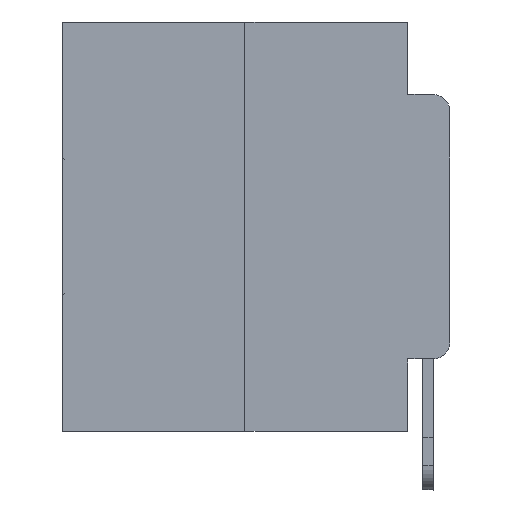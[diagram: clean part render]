
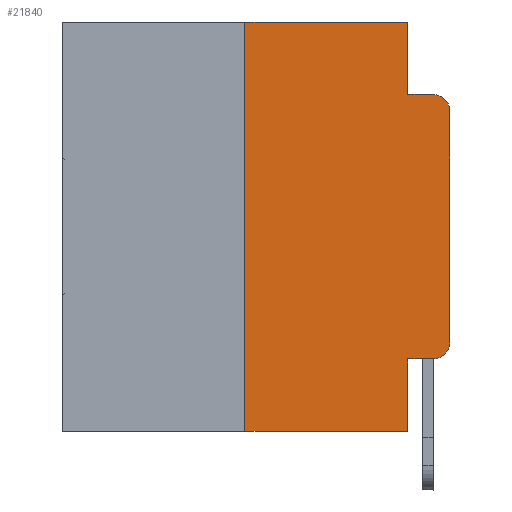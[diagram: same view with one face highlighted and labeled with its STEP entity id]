
A CAD part, left-side view. The second image highlights one B-rep face of the part: STEP entity #21840.
In plain terms, the highlighted planar face has unit normal (-1, 0, 0).
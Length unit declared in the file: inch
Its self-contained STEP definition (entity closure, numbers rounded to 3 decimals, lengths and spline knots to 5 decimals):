
#330 = VECTOR ( 'NONE', #6012, 39.37008 ) ;
#424 = VERTEX_POINT ( 'NONE', #10604 ) ;
#561 = VERTEX_POINT ( 'NONE', #18471 ) ;
#681 = EDGE_CURVE ( 'NONE', #25812, #13251, #2712, .T. ) ;
#695 = DIRECTION ( 'NONE',  ( 0., 0., -1. ) ) ;
#909 = CARTESIAN_POINT ( 'NONE',  ( 0., 0.25, -0.5 ) ) ;
#973 = LINE ( 'NONE', #10256, #26349 ) ;
#981 = EDGE_CURVE ( 'NONE', #2147, #25812, #7429, .T. ) ;
#996 = CARTESIAN_POINT ( 'NONE',  ( 0., 0.051, 0. ) ) ;
#1854 = CARTESIAN_POINT ( 'NONE',  ( 0., 0.02, -0.3915 ) ) ;
#2147 = VERTEX_POINT ( 'NONE', #7585 ) ;
#2471 = CIRCLE ( 'NONE', #28664, 0.02 ) ;
#2712 = CIRCLE ( 'NONE', #18216, 0.02 ) ;
#2861 = CARTESIAN_POINT ( 'NONE',  ( 0., 0., 0. ) ) ;
#2987 = CARTESIAN_POINT ( 'NONE',  ( 0., 0.02, -0.1085 ) ) ;
#2998 = DIRECTION ( 'NONE',  ( 0., 0., -1. ) ) ;
#3108 = PLANE ( 'NONE',  #6923 ) ;
#3153 = CARTESIAN_POINT ( 'NONE',  ( 0., 0.051, -0.0885 ) ) ;
#4229 = ORIENTED_EDGE ( 'NONE', *, *, #6345, .T. ) ;
#4596 = DIRECTION ( 'NONE',  ( 0., -1., 0. ) ) ;
#4741 = ORIENTED_EDGE ( 'NONE', *, *, #19063, .F. ) ;
#5782 = EDGE_CURVE ( 'NONE', #561, #13251, #15111, .T. ) ;
#5918 = CARTESIAN_POINT ( 'NONE',  ( 0., 0., -0.1085 ) ) ;
#6012 = DIRECTION ( 'NONE',  ( 0., -1., 0. ) ) ;
#6345 = EDGE_CURVE ( 'NONE', #14868, #16988, #973, .T. ) ;
#6880 = LINE ( 'NONE', #20534, #29394 ) ;
#6923 = AXIS2_PLACEMENT_3D ( 'NONE', #15220, #17502, #12649 ) ;
#7281 = EDGE_CURVE ( 'NONE', #14868, #12450, #22466, .T. ) ;
#7429 = LINE ( 'NONE', #2861, #10027 ) ;
#7585 = CARTESIAN_POINT ( 'NONE',  ( 0., 0., -0.3915 ) ) ;
#8486 = ORIENTED_EDGE ( 'NONE', *, *, #681, .T. ) ;
#9009 = DIRECTION ( 'NONE',  ( 0., 0., -1. ) ) ;
#9286 = VERTEX_POINT ( 'NONE', #29102 ) ;
#9559 = DIRECTION ( 'NONE',  ( 0., 0., 1. ) ) ;
#9610 = VERTEX_POINT ( 'NONE', #18593 ) ;
#9802 = LINE ( 'NONE', #28182, #21337 ) ;
#10027 = VECTOR ( 'NONE', #9559, 39.37008 ) ;
#10256 = CARTESIAN_POINT ( 'NONE',  ( 0., 0.473, -0.5 ) ) ;
#10604 = CARTESIAN_POINT ( 'NONE',  ( 0., 0.051, 0. ) ) ;
#12450 = VERTEX_POINT ( 'NONE', #28972 ) ;
#12649 = DIRECTION ( 'NONE',  ( 0., 0., -1. ) ) ;
#13251 = VERTEX_POINT ( 'NONE', #25727 ) ;
#14868 = VERTEX_POINT ( 'NONE', #909 ) ;
#15111 = LINE ( 'NONE', #3153, #330 ) ;
#15220 = CARTESIAN_POINT ( 'NONE',  ( 0., 0.473, 0. ) ) ;
#15314 = DIRECTION ( 'NONE',  ( 0., 0., 1. ) ) ;
#15865 = EDGE_CURVE ( 'NONE', #9286, #2147, #2471, .T. ) ;
#15973 = ORIENTED_EDGE ( 'NONE', *, *, #5782, .F. ) ;
#16988 = VERTEX_POINT ( 'NONE', #24145 ) ;
#17148 = ORIENTED_EDGE ( 'NONE', *, *, #18655, .F. ) ;
#17150 = EDGE_LOOP ( 'NONE', ( #24414, #8486, #15973, #29195, #4741, #17432, #4229, #17148, #26818, #22518 ) ) ;
#17432 = ORIENTED_EDGE ( 'NONE', *, *, #7281, .F. ) ;
#17502 = DIRECTION ( 'NONE',  ( 1., 0., 0. ) ) ;
#17875 = LINE ( 'NONE', #27167, #27758 ) ;
#18216 = AXIS2_PLACEMENT_3D ( 'NONE', #2987, #21362, #695 ) ;
#18393 = VECTOR ( 'NONE', #2998, 39.37008 ) ;
#18399 = EDGE_CURVE ( 'NONE', #424, #561, #17875, .T. ) ;
#18471 = CARTESIAN_POINT ( 'NONE',  ( 0., 0.051, -0.0885 ) ) ;
#18593 = CARTESIAN_POINT ( 'NONE',  ( 0., 0.051, -0.4115 ) ) ;
#18655 = EDGE_CURVE ( 'NONE', #9610, #16988, #28659, .T. ) ;
#19063 = EDGE_CURVE ( 'NONE', #12450, #424, #9802, .T. ) ;
#20534 = CARTESIAN_POINT ( 'NONE',  ( 0., 0.051, -0.4115 ) ) ;
#21337 = VECTOR ( 'NONE', #23636, 39.37008 ) ;
#21362 = DIRECTION ( 'NONE',  ( -1., 0., 0. ) ) ;
#21840 = ADVANCED_FACE ( 'NONE', ( #24221 ), #3108, .F. ) ;
#22466 = LINE ( 'NONE', #26734, #28799 ) ;
#22518 = ORIENTED_EDGE ( 'NONE', *, *, #15865, .T. ) ;
#23636 = DIRECTION ( 'NONE',  ( 0., -1., 0. ) ) ;
#24145 = CARTESIAN_POINT ( 'NONE',  ( 0., 0.051, -0.5 ) ) ;
#24221 = FACE_OUTER_BOUND ( 'NONE', #17150, .T. ) ;
#24414 = ORIENTED_EDGE ( 'NONE', *, *, #981, .T. ) ;
#25727 = CARTESIAN_POINT ( 'NONE',  ( 0., 0.02, -0.0885 ) ) ;
#25812 = VERTEX_POINT ( 'NONE', #5918 ) ;
#26209 = DIRECTION ( 'NONE',  ( 0., -1., 0. ) ) ;
#26349 = VECTOR ( 'NONE', #26209, 39.37008 ) ;
#26734 = CARTESIAN_POINT ( 'NONE',  ( 0., 0.25, 0. ) ) ;
#26764 = EDGE_CURVE ( 'NONE', #9610, #9286, #6880, .T. ) ;
#26818 = ORIENTED_EDGE ( 'NONE', *, *, #26764, .T. ) ;
#27167 = CARTESIAN_POINT ( 'NONE',  ( 0., 0.051, 0. ) ) ;
#27537 = DIRECTION ( 'NONE',  ( -1., 0., 0. ) ) ;
#27758 = VECTOR ( 'NONE', #29143, 39.37008 ) ;
#28182 = CARTESIAN_POINT ( 'NONE',  ( 0., 0.473, 0. ) ) ;
#28659 = LINE ( 'NONE', #996, #18393 ) ;
#28664 = AXIS2_PLACEMENT_3D ( 'NONE', #1854, #27537, #9009 ) ;
#28799 = VECTOR ( 'NONE', #15314, 39.37008 ) ;
#28972 = CARTESIAN_POINT ( 'NONE',  ( 0., 0.25, 0. ) ) ;
#29102 = CARTESIAN_POINT ( 'NONE',  ( 0., 0.02, -0.4115 ) ) ;
#29143 = DIRECTION ( 'NONE',  ( 0., 0., -1. ) ) ;
#29195 = ORIENTED_EDGE ( 'NONE', *, *, #18399, .F. ) ;
#29394 = VECTOR ( 'NONE', #4596, 39.37008 ) ;
